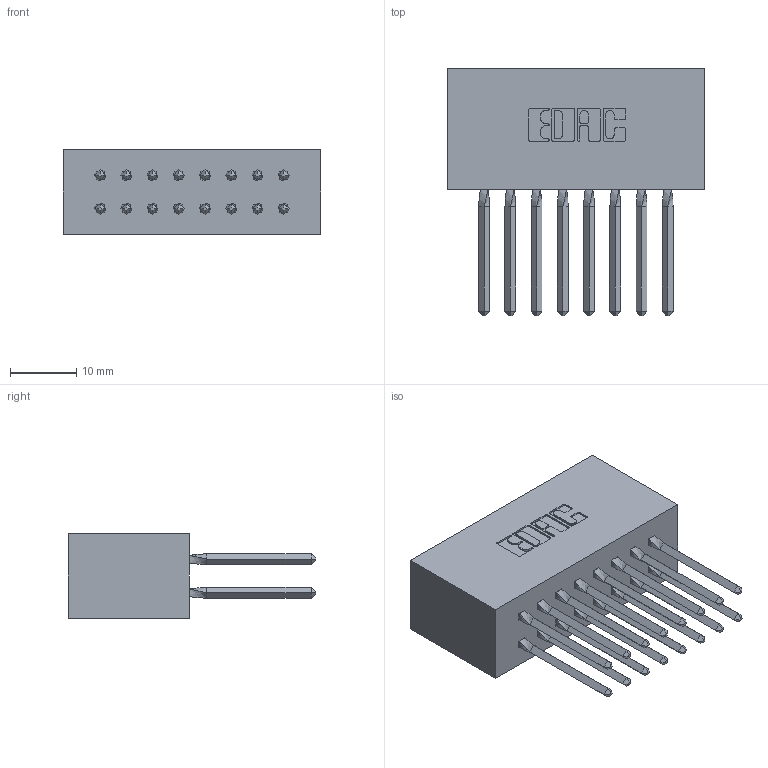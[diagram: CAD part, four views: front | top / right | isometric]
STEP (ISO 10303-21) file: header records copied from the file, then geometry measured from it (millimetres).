
FILE_DESCRIPTION (( 'STEP AP203' ), '1' );
FILE_NAME ('317-016-540-801.STEP', '2020-02-27T15:18:55', ( '' ), ( '' ), 'SwSTEP 2.0', 'SolidWorks 2016', '' );
FILE_SCHEMA (( 'CONFIG_CONTROL_DESIGN' ));
Length unit declared in the file: inch
Products named in the file (3): 317 Part_Lugless; 317-016-540-801; 317-290-001_540
Assembly tree (17 placements, depth 2):
  317-016-540-801
    317 Part_Lugless
    317-290-001_540  x16
Bounding box: 38.91 x 37.34 x 12.7 mm (x, y, z)
Volume: 7174.8 mm3; surface area: 9669.3 mm2
Topology: 17 solids, 17 shells, 1514 faces, 4191 edges, 2702 vertices
Faces by surface type: plane 1218, cylinder 232, bspline 64
Entity records: 15898 total; most frequent: CARTESIAN_POINT 3183, ORIENTED_EDGE 2682, DIRECTION 2235, EDGE_CURVE 1341, VECTOR 1093, LINE 1093, VERTEX_POINT 887, AXIS2_PLACEMENT_3D 571
